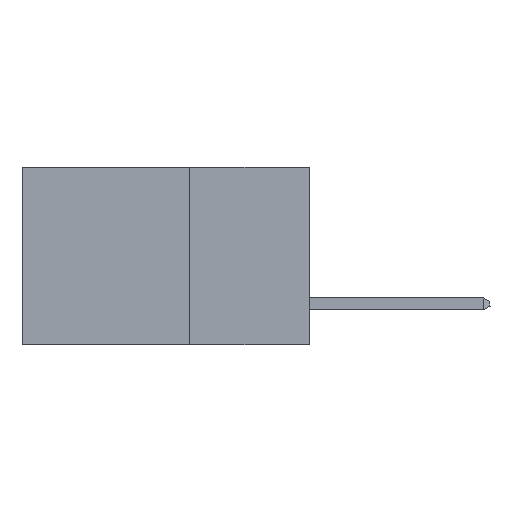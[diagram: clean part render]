
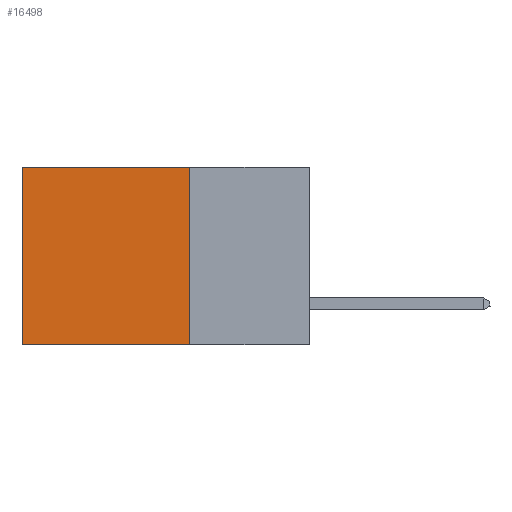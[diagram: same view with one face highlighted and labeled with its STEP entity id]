
A CAD part, left-side view. The second image highlights one B-rep face of the part: STEP entity #16498.
In plain terms, the highlighted planar face has unit normal (-1, 0, 0).
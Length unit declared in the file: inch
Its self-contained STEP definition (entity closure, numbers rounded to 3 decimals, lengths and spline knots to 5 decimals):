
#113 = LINE ( 'NONE', #468, #17060 ) ;
#468 = CARTESIAN_POINT ( 'NONE',  ( 0.2875, 0.25, 0. ) ) ;
#850 = ORIENTED_EDGE ( 'NONE', *, *, #8300, .F. ) ;
#1656 = CARTESIAN_POINT ( 'NONE',  ( 0.2875, 0.25, 0. ) ) ;
#1960 = EDGE_CURVE ( 'NONE', #12886, #11093, #4045, .T. ) ;
#2130 = DIRECTION ( 'NONE',  ( 0., 0., -1. ) ) ;
#2597 = ORIENTED_EDGE ( 'NONE', *, *, #15958, .F. ) ;
#2925 = FACE_OUTER_BOUND ( 'NONE', #16541, .T. ) ;
#3388 = CARTESIAN_POINT ( 'NONE',  ( 0.2875, 0.25, 0. ) ) ;
#4045 = LINE ( 'NONE', #10008, #20253 ) ;
#5106 = PLANE ( 'NONE',  #15312 ) ;
#5514 = VECTOR ( 'NONE', #15946, 39.37008 ) ;
#5586 = VERTEX_POINT ( 'NONE', #14151 ) ;
#5660 = EDGE_CURVE ( 'NONE', #5586, #12886, #9728, .T. ) ;
#6728 = DIRECTION ( 'NONE',  ( 0., 0., -1. ) ) ;
#7228 = CARTESIAN_POINT ( 'NONE',  ( 0.2875, 0.6, 0. ) ) ;
#7296 = CARTESIAN_POINT ( 'NONE',  ( 0.2875, 0.25, -0.37 ) ) ;
#7438 = VECTOR ( 'NONE', #11796, 39.37008 ) ;
#8300 = EDGE_CURVE ( 'NONE', #16746, #11093, #12068, .T. ) ;
#8724 = ORIENTED_EDGE ( 'NONE', *, *, #1960, .T. ) ;
#9728 = LINE ( 'NONE', #1656, #5514 ) ;
#9841 = DIRECTION ( 'NONE',  ( 0., 0., -1. ) ) ;
#10008 = CARTESIAN_POINT ( 'NONE',  ( 0.2875, 0.6, 0. ) ) ;
#11093 = VERTEX_POINT ( 'NONE', #18417 ) ;
#11796 = DIRECTION ( 'NONE',  ( 0., 1., 0. ) ) ;
#12068 = LINE ( 'NONE', #14922, #7438 ) ;
#12401 = ORIENTED_EDGE ( 'NONE', *, *, #5660, .T. ) ;
#12886 = VERTEX_POINT ( 'NONE', #7228 ) ;
#14151 = CARTESIAN_POINT ( 'NONE',  ( 0.2875, 0.25, 0. ) ) ;
#14922 = CARTESIAN_POINT ( 'NONE',  ( 0.2875, 0.25, -0.37 ) ) ;
#15312 = AXIS2_PLACEMENT_3D ( 'NONE', #3388, #16129, #6728 ) ;
#15946 = DIRECTION ( 'NONE',  ( 0., 1., 0. ) ) ;
#15958 = EDGE_CURVE ( 'NONE', #5586, #16746, #113, .T. ) ;
#16129 = DIRECTION ( 'NONE',  ( 1., 0., 0. ) ) ;
#16498 = ADVANCED_FACE ( 'NONE', ( #2925 ), #5106, .F. ) ;
#16541 = EDGE_LOOP ( 'NONE', ( #8724, #850, #2597, #12401 ) ) ;
#16746 = VERTEX_POINT ( 'NONE', #7296 ) ;
#17060 = VECTOR ( 'NONE', #2130, 39.37008 ) ;
#18417 = CARTESIAN_POINT ( 'NONE',  ( 0.2875, 0.6, -0.37 ) ) ;
#20253 = VECTOR ( 'NONE', #9841, 39.37008 ) ;
